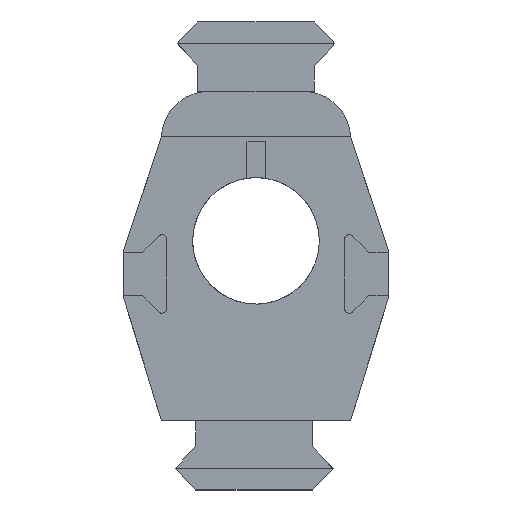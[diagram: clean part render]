
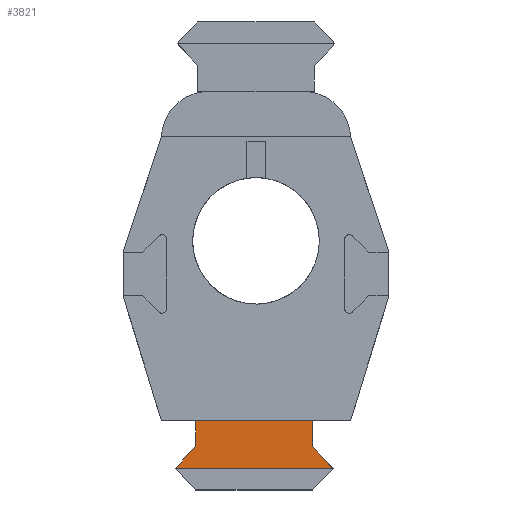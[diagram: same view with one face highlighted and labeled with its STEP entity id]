
A CAD part, front view. The second image highlights one B-rep face of the part: STEP entity #3821.
In plain terms, the highlighted planar face has unit normal (0, -1, 0).
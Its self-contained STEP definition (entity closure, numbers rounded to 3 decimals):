
#192=FACE_OUTER_BOUND('',#405,.T.);
#405=EDGE_LOOP('',(#2957,#2958,#2959,#2960,#2961,#2962));
#752=LINE('',#5822,#1257);
#753=LINE('',#5825,#1258);
#754=LINE('',#5827,#1259);
#755=LINE('',#5829,#1260);
#756=LINE('',#5831,#1261);
#757=LINE('',#5832,#1262);
#1257=VECTOR('',#4710,10.);
#1258=VECTOR('',#4713,10.);
#1259=VECTOR('',#4714,10.);
#1260=VECTOR('',#4715,10.);
#1261=VECTOR('',#4716,10.);
#1262=VECTOR('',#4717,10.);
#1690=VERTEX_POINT('',#5747);
#1727=VERTEX_POINT('',#5820);
#1728=VERTEX_POINT('',#5824);
#1729=VERTEX_POINT('',#5826);
#1730=VERTEX_POINT('',#5828);
#1731=VERTEX_POINT('',#5830);
#2164=EDGE_CURVE('',#1727,#1690,#752,.T.);
#2165=EDGE_CURVE('',#1728,#1727,#753,.T.);
#2166=EDGE_CURVE('',#1729,#1728,#754,.T.);
#2167=EDGE_CURVE('',#1730,#1729,#755,.T.);
#2168=EDGE_CURVE('',#1731,#1730,#756,.T.);
#2169=EDGE_CURVE('',#1690,#1731,#757,.T.);
#2957=ORIENTED_EDGE('',*,*,#2165,.F.);
#2958=ORIENTED_EDGE('',*,*,#2166,.F.);
#2959=ORIENTED_EDGE('',*,*,#2167,.F.);
#2960=ORIENTED_EDGE('',*,*,#2168,.F.);
#2961=ORIENTED_EDGE('',*,*,#2169,.F.);
#2962=ORIENTED_EDGE('',*,*,#2164,.F.);
#3612=PLANE('',#4093);
#3821=ADVANCED_FACE('',(#192),#3612,.F.);
#4093=AXIS2_PLACEMENT_3D('',#5823,#4711,#4712);
#4710=DIRECTION('',(0.691,0.,-0.723));
#4711=DIRECTION('center_axis',(0.,1.,0.));
#4712=DIRECTION('ref_axis',(0.,0.,1.));
#4713=DIRECTION('',(0.,0.,-1.));
#4714=DIRECTION('',(1.,0.,0.));
#4715=DIRECTION('',(0.,0.,1.));
#4716=DIRECTION('',(0.689,0.,0.725));
#4717=DIRECTION('',(-1.,0.,0.));
#5747=CARTESIAN_POINT('',(10.321,171.04,-19.102));
#5820=CARTESIAN_POINT('',(7.582,171.04,-16.235));
#5822=CARTESIAN_POINT('',(6.671,171.04,-15.282));
#5823=CARTESIAN_POINT('Origin',(-8.09,171.04,-22.022));
#5824=CARTESIAN_POINT('',(7.582,171.04,-12.7));
#5825=CARTESIAN_POINT('',(7.582,171.04,-19.129));
#5826=CARTESIAN_POINT('',(-8.09,171.04,-12.7));
#5827=CARTESIAN_POINT('',(-0.254,171.04,-12.7));
#5828=CARTESIAN_POINT('',(-8.09,171.04,-16.19));
#5829=CARTESIAN_POINT('',(-8.09,171.04,-17.361));
#5830=CARTESIAN_POINT('',(-10.858,171.04,-19.102));
#5831=CARTESIAN_POINT('',(-9.546,171.04,-17.721));
#5832=CARTESIAN_POINT('',(-8.09,171.04,-19.102));
